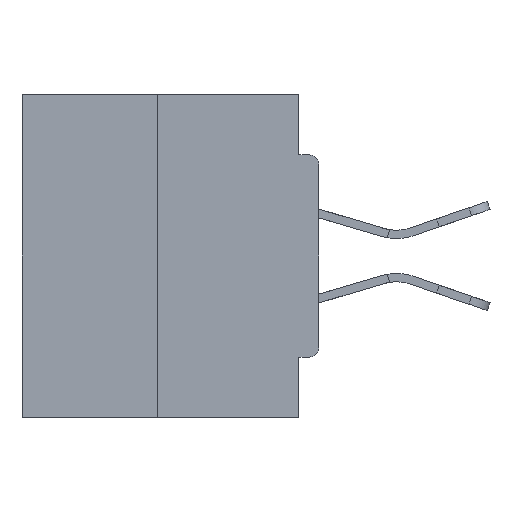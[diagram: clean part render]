
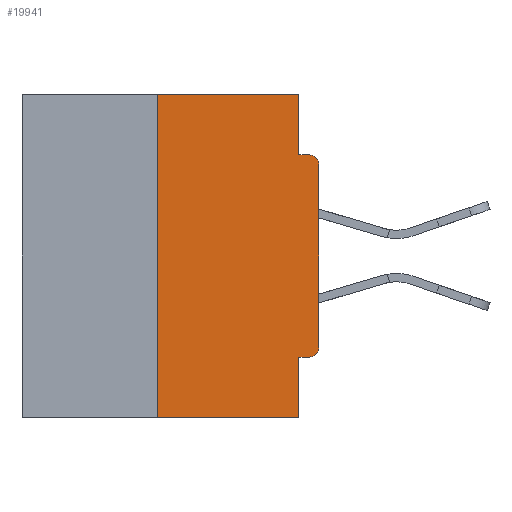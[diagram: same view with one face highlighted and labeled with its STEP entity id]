
A CAD part, left-side view. The second image highlights one B-rep face of the part: STEP entity #19941.
In plain terms, the highlighted planar face has unit normal (-1, 0, 0).
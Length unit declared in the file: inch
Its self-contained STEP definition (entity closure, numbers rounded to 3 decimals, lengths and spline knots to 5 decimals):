
#332 = VERTEX_POINT ( 'NONE', #25613 ) ;
#615 = EDGE_CURVE ( 'NONE', #23482, #9055, #14059, .T. ) ;
#1536 = CARTESIAN_POINT ( 'NONE',  ( 0., 0.015, -0.0935 ) ) ;
#1653 = AXIS2_PLACEMENT_3D ( 'NONE', #3904, #21669, #3773 ) ;
#2185 = ORIENTED_EDGE ( 'NONE', *, *, #27704, .T. ) ;
#2213 = DIRECTION ( 'NONE',  ( 0., 0., -1. ) ) ;
#2345 = CARTESIAN_POINT ( 'NONE',  ( 0., 0., 0. ) ) ;
#2512 = DIRECTION ( 'NONE',  ( 0., 0., 1. ) ) ;
#3713 = EDGE_CURVE ( 'NONE', #23592, #16954, #7448, .T. ) ;
#3773 = DIRECTION ( 'NONE',  ( 0., 0., -1. ) ) ;
#3813 = EDGE_CURVE ( 'NONE', #23482, #8968, #4666, .T. ) ;
#3904 = CARTESIAN_POINT ( 'NONE',  ( 0., 0.015, -0.3915 ) ) ;
#4045 = VERTEX_POINT ( 'NONE', #34204 ) ;
#4420 = VECTOR ( 'NONE', #9433, 39.37008 ) ;
#4526 = CARTESIAN_POINT ( 'NONE',  ( 0., 0.25, 0. ) ) ;
#4666 = CIRCLE ( 'NONE', #1653, 0.015 ) ;
#4670 = CARTESIAN_POINT ( 'NONE',  ( 0., 0.031, -0.4065 ) ) ;
#4801 = ORIENTED_EDGE ( 'NONE', *, *, #3813, .T. ) ;
#5739 = LINE ( 'NONE', #10931, #23942 ) ;
#5805 = CARTESIAN_POINT ( 'NONE',  ( 0., 0.25, 0. ) ) ;
#6026 = ORIENTED_EDGE ( 'NONE', *, *, #33441, .T. ) ;
#6491 = VECTOR ( 'NONE', #7671, 39.37008 ) ;
#7431 = EDGE_CURVE ( 'NONE', #4045, #27814, #25338, .T. ) ;
#7448 = LINE ( 'NONE', #5805, #36506 ) ;
#7671 = DIRECTION ( 'NONE',  ( 0., -1., 0. ) ) ;
#8348 = CARTESIAN_POINT ( 'NONE',  ( 0., 0.46, 0. ) ) ;
#8564 = CIRCLE ( 'NONE', #18591, 0.015 ) ;
#8595 = DIRECTION ( 'NONE',  ( 0., 0., -1. ) ) ;
#8968 = VERTEX_POINT ( 'NONE', #25462 ) ;
#9055 = VERTEX_POINT ( 'NONE', #4670 ) ;
#9433 = DIRECTION ( 'NONE',  ( 0., -1., 0. ) ) ;
#9943 = VECTOR ( 'NONE', #8595, 39.37008 ) ;
#10931 = CARTESIAN_POINT ( 'NONE',  ( 0., 0.46, -0.5 ) ) ;
#12012 = DIRECTION ( 'NONE',  ( 0., 0., -1. ) ) ;
#12865 = ORIENTED_EDGE ( 'NONE', *, *, #36240, .F. ) ;
#13158 = ORIENTED_EDGE ( 'NONE', *, *, #615, .F. ) ;
#13975 = DIRECTION ( 'NONE',  ( 0., -1., 0. ) ) ;
#14059 = LINE ( 'NONE', #35633, #28575 ) ;
#14088 = ORIENTED_EDGE ( 'NONE', *, *, #18532, .F. ) ;
#16954 = VERTEX_POINT ( 'NONE', #4526 ) ;
#17007 = DIRECTION ( 'NONE',  ( 0., 0., 1. ) ) ;
#18532 = EDGE_CURVE ( 'NONE', #27814, #34375, #27425, .T. ) ;
#18591 = AXIS2_PLACEMENT_3D ( 'NONE', #32161, #35308, #12012 ) ;
#19651 = CARTESIAN_POINT ( 'NONE',  ( 0., 0.031, -0.5 ) ) ;
#19782 = DIRECTION ( 'NONE',  ( 0., 0., -1. ) ) ;
#19941 = ADVANCED_FACE ( 'NONE', ( #29547 ), #37033, .F. ) ;
#20314 = AXIS2_PLACEMENT_3D ( 'NONE', #8348, #37150, #19782 ) ;
#20916 = CARTESIAN_POINT ( 'NONE',  ( 0., 0.25, -0.5 ) ) ;
#21233 = CARTESIAN_POINT ( 'NONE',  ( 0., 0.46, 0. ) ) ;
#21309 = DIRECTION ( 'NONE',  ( 0., 1., 0. ) ) ;
#21669 = DIRECTION ( 'NONE',  ( -1., 0., 0. ) ) ;
#22299 = CARTESIAN_POINT ( 'NONE',  ( 0., 0.031, -0.0935 ) ) ;
#22801 = LINE ( 'NONE', #2345, #32820 ) ;
#23133 = VECTOR ( 'NONE', #2213, 39.37008 ) ;
#23482 = VERTEX_POINT ( 'NONE', #28644 ) ;
#23592 = VERTEX_POINT ( 'NONE', #20916 ) ;
#23942 = VECTOR ( 'NONE', #13975, 39.37008 ) ;
#25097 = EDGE_CURVE ( 'NONE', #23592, #27861, #5739, .T. ) ;
#25338 = LINE ( 'NONE', #25990, #9943 ) ;
#25462 = CARTESIAN_POINT ( 'NONE',  ( 0., 0., -0.3915 ) ) ;
#25613 = CARTESIAN_POINT ( 'NONE',  ( 0., 0., -0.1085 ) ) ;
#25990 = CARTESIAN_POINT ( 'NONE',  ( 0., 0.031, 0. ) ) ;
#26048 = ORIENTED_EDGE ( 'NONE', *, *, #25097, .T. ) ;
#27425 = LINE ( 'NONE', #33439, #6491 ) ;
#27704 = EDGE_CURVE ( 'NONE', #8968, #332, #22801, .T. ) ;
#27814 = VERTEX_POINT ( 'NONE', #22299 ) ;
#27861 = VERTEX_POINT ( 'NONE', #37277 ) ;
#28575 = VECTOR ( 'NONE', #21309, 39.37008 ) ;
#28644 = CARTESIAN_POINT ( 'NONE',  ( 0., 0.015, -0.4065 ) ) ;
#29547 = FACE_OUTER_BOUND ( 'NONE', #30250, .T. ) ;
#30250 = EDGE_LOOP ( 'NONE', ( #12865, #30500, #26048, #31891, #13158, #4801, #2185, #6026, #14088, #35952 ) ) ;
#30500 = ORIENTED_EDGE ( 'NONE', *, *, #3713, .F. ) ;
#30845 = LINE ( 'NONE', #19651, #23133 ) ;
#31891 = ORIENTED_EDGE ( 'NONE', *, *, #33108, .F. ) ;
#32161 = CARTESIAN_POINT ( 'NONE',  ( 0., 0.015, -0.1085 ) ) ;
#32600 = LINE ( 'NONE', #21233, #4420 ) ;
#32820 = VECTOR ( 'NONE', #17007, 39.37008 ) ;
#33108 = EDGE_CURVE ( 'NONE', #9055, #27861, #30845, .T. ) ;
#33439 = CARTESIAN_POINT ( 'NONE',  ( 0., 0., -0.0935 ) ) ;
#33441 = EDGE_CURVE ( 'NONE', #332, #34375, #8564, .T. ) ;
#34204 = CARTESIAN_POINT ( 'NONE',  ( 0., 0.031, 0. ) ) ;
#34375 = VERTEX_POINT ( 'NONE', #1536 ) ;
#35308 = DIRECTION ( 'NONE',  ( -1., 0., 0. ) ) ;
#35633 = CARTESIAN_POINT ( 'NONE',  ( 0., 0., -0.4065 ) ) ;
#35952 = ORIENTED_EDGE ( 'NONE', *, *, #7431, .F. ) ;
#36240 = EDGE_CURVE ( 'NONE', #16954, #4045, #32600, .T. ) ;
#36506 = VECTOR ( 'NONE', #2512, 39.37008 ) ;
#37033 = PLANE ( 'NONE',  #20314 ) ;
#37150 = DIRECTION ( 'NONE',  ( 1., 0., 0. ) ) ;
#37277 = CARTESIAN_POINT ( 'NONE',  ( 0., 0.031, -0.5 ) ) ;
